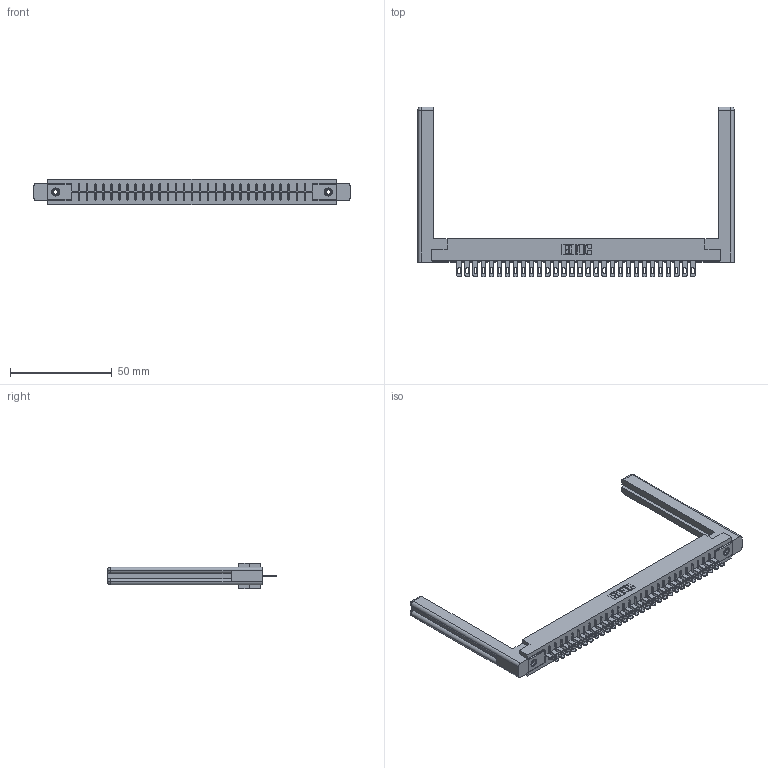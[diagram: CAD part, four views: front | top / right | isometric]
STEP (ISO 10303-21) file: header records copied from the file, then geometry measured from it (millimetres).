
FILE_DESCRIPTION (( 'STEP AP203' ), '1' );
FILE_NAME ('306-030-500-158.STEP', '2019-09-11T22:19:31', ( '' ), ( '' ), 'SwSTEP 2.0', 'SolidWorks 2016', '' );
FILE_SCHEMA (( 'CONFIG_CONTROL_DESIGN' ));
Length unit declared in the file: inch
Products named in the file (5): 306-030-500-158; 306-290-001_100; 306 Part_.156 Dia; 307-220-058; 345-250-001_345-250-001-102
Assembly tree (35 placements, depth 2):
  306-030-500-158
    306 Part_.156 Dia
    306-290-001_100  x30
    345-250-001_345-250-001-102  x2
    307-220-058  x2
Bounding box: 155.5 x 83.52 x 12.7 mm (x, y, z)
Volume: 24252.1 mm3; surface area: 23160.7 mm2
Topology: 35 solids, 35 shells, 2538 faces, 7120 edges, 4572 vertices
Faces by surface type: plane 1652, cylinder 742, sphere 120, cone 12, torus 12
Entity records: 32328 total; most frequent: CARTESIAN_POINT 5436, ORIENTED_EDGE 5330, DIRECTION 5317, EDGE_CURVE 2665, VECTOR 2071, LINE 2071, VERTEX_POINT 1688, AXIS2_PLACEMENT_3D 1623
